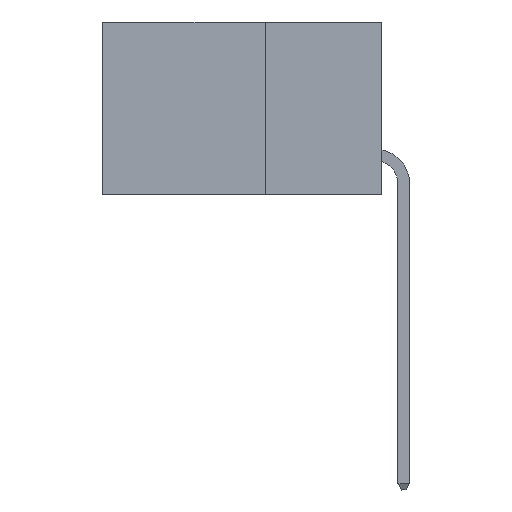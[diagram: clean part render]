
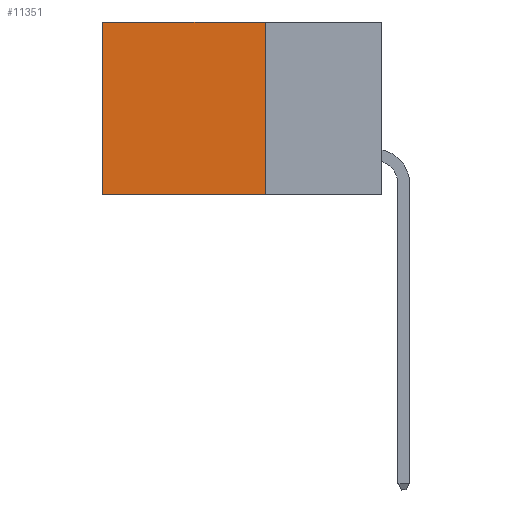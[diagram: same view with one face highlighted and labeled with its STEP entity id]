
A CAD part, left-side view. The second image highlights one B-rep face of the part: STEP entity #11351.
In plain terms, the highlighted planar face has unit normal (-1, 0, 0).
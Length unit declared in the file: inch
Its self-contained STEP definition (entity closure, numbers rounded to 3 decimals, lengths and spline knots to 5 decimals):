
#2129 = EDGE_CURVE ( 'NONE', #17424, #13507, #37676, .T. ) ;
#3559 = ORIENTED_EDGE ( 'NONE', *, *, #10788, .T. ) ;
#4269 = ORIENTED_EDGE ( 'NONE', *, *, #9276, .T. ) ;
#5351 = VECTOR ( 'NONE', #20642, 39.37008 ) ;
#6244 = DIRECTION ( 'NONE',  ( 0., 1., 0. ) ) ;
#6727 = FACE_OUTER_BOUND ( 'NONE', #20496, .T. ) ;
#7064 = ORIENTED_EDGE ( 'NONE', *, *, #26200, .F. ) ;
#7649 = VERTEX_POINT ( 'NONE', #26781 ) ;
#9276 = EDGE_CURVE ( 'NONE', #17424, #31767, #9667, .T. ) ;
#9667 = LINE ( 'NONE', #34695, #26662 ) ;
#10788 = EDGE_CURVE ( 'NONE', #31767, #7649, #14807, .T. ) ;
#11351 = ADVANCED_FACE ( 'NONE', ( #6727 ), #21411, .F. ) ;
#12325 = CARTESIAN_POINT ( 'NONE',  ( 0.2875, 0.25, 0. ) ) ;
#13052 = CARTESIAN_POINT ( 'NONE',  ( 0.2875, 0.25, 0. ) ) ;
#13403 = LINE ( 'NONE', #33053, #24683 ) ;
#13507 = VERTEX_POINT ( 'NONE', #15843 ) ;
#13785 = CARTESIAN_POINT ( 'NONE',  ( 0.2875, 0.6, 0. ) ) ;
#14807 = LINE ( 'NONE', #13785, #5351 ) ;
#15843 = CARTESIAN_POINT ( 'NONE',  ( 0.2875, 0.25, -0.37 ) ) ;
#16614 = DIRECTION ( 'NONE',  ( 0., 1., 0. ) ) ;
#17424 = VERTEX_POINT ( 'NONE', #13052 ) ;
#17731 = ORIENTED_EDGE ( 'NONE', *, *, #2129, .F. ) ;
#20496 = EDGE_LOOP ( 'NONE', ( #3559, #7064, #17731, #4269 ) ) ;
#20642 = DIRECTION ( 'NONE',  ( 0., 0., -1. ) ) ;
#21360 = AXIS2_PLACEMENT_3D ( 'NONE', #12325, #33444, #36452 ) ;
#21411 = PLANE ( 'NONE',  #21360 ) ;
#23322 = CARTESIAN_POINT ( 'NONE',  ( 0.2875, 0.6, 0. ) ) ;
#24683 = VECTOR ( 'NONE', #6244, 39.37008 ) ;
#26200 = EDGE_CURVE ( 'NONE', #13507, #7649, #13403, .T. ) ;
#26662 = VECTOR ( 'NONE', #16614, 39.37008 ) ;
#26781 = CARTESIAN_POINT ( 'NONE',  ( 0.2875, 0.6, -0.37 ) ) ;
#29924 = DIRECTION ( 'NONE',  ( 0., 0., -1. ) ) ;
#31767 = VERTEX_POINT ( 'NONE', #23322 ) ;
#32965 = VECTOR ( 'NONE', #29924, 39.37008 ) ;
#33053 = CARTESIAN_POINT ( 'NONE',  ( 0.2875, 0.25, -0.37 ) ) ;
#33444 = DIRECTION ( 'NONE',  ( 1., 0., 0. ) ) ;
#34695 = CARTESIAN_POINT ( 'NONE',  ( 0.2875, 0.25, 0. ) ) ;
#35205 = CARTESIAN_POINT ( 'NONE',  ( 0.2875, 0.25, 0. ) ) ;
#36452 = DIRECTION ( 'NONE',  ( 0., 0., -1. ) ) ;
#37676 = LINE ( 'NONE', #35205, #32965 ) ;
